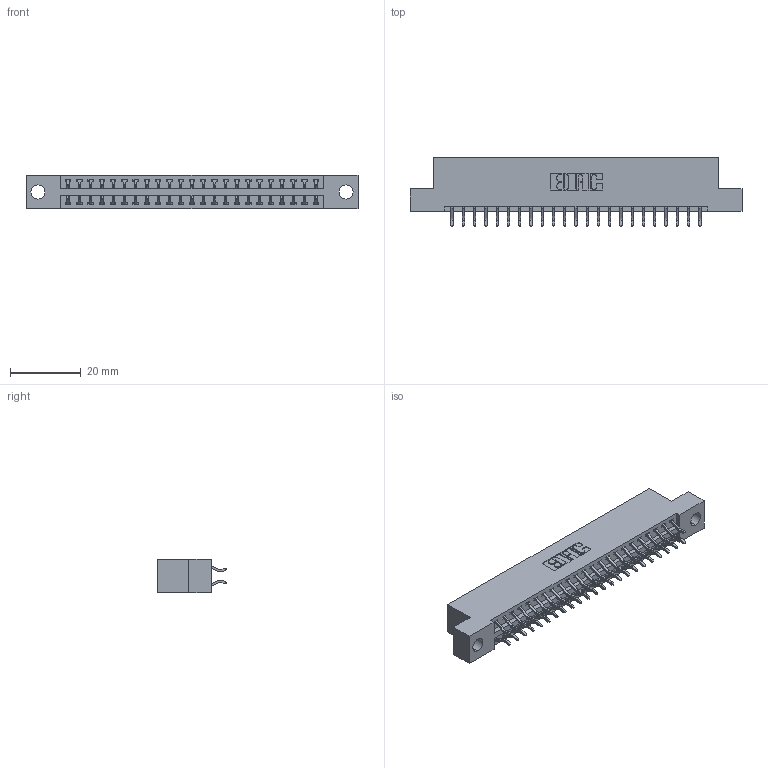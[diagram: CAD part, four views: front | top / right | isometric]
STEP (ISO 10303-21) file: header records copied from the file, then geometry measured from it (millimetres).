
FILE_DESCRIPTION (( 'STEP AP203' ), '1' );
FILE_NAME ('346-046-556-204.STEP', '2022-05-20T20:20:18', ( '' ), ( '' ), 'SwSTEP 2.0', 'SolidWorks 2020', '' );
FILE_SCHEMA (( 'CONFIG_CONTROL_DESIGN' ));
Length unit declared in the file: inch
Products named in the file (3): 346 Part_Flush Mounting Lugs - 0.156 Dia-TH; 345-292-001_556 Tail; 346-046-556-204
Assembly tree (47 placements, depth 2):
  346-046-556-204
    346 Part_Flush Mounting Lugs - 0.156 Dia-TH
    345-292-001_556 Tail  x46
Bounding box: 93.6 x 19.57 x 9.4 mm (x, y, z)
Volume: 8871.7 mm3; surface area: 11701.3 mm2
Topology: 47 solids, 47 shells, 2804 faces, 8323 edges, 5486 vertices
Faces by surface type: plane 1884, cylinder 920
Entity records: 18207 total; most frequent: CARTESIAN_POINT 3046, ORIENTED_EDGE 2966, DIRECTION 2723, EDGE_CURVE 1483, LINE 1251, VECTOR 1251, VERTEX_POINT 986, AXIS2_PLACEMENT_3D 736
